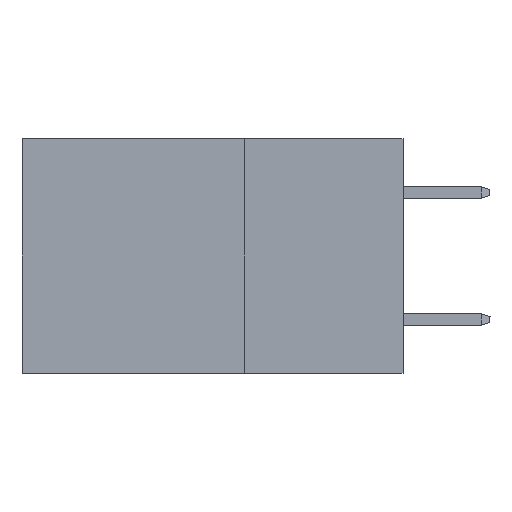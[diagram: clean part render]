
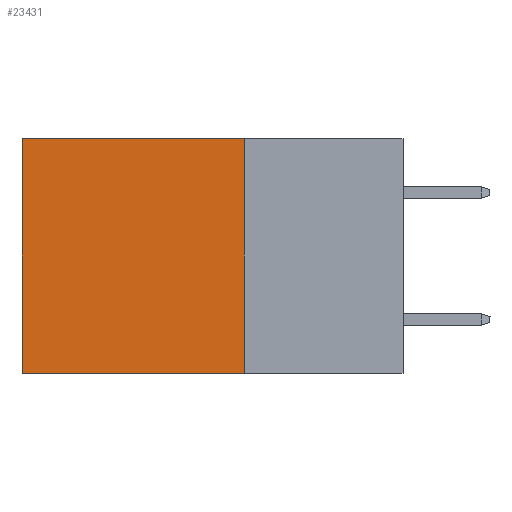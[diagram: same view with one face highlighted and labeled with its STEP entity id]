
A CAD part, left-side view. The second image highlights one B-rep face of the part: STEP entity #23431.
In plain terms, the highlighted planar face has unit normal (-1, 0, 0).
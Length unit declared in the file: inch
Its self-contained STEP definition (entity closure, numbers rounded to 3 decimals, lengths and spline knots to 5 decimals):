
#211 = ORIENTED_EDGE ( 'NONE', *, *, #19550, .T. ) ;
#2471 = DIRECTION ( 'NONE',  ( 0., 0., -1. ) ) ;
#2619 = EDGE_CURVE ( 'NONE', #22974, #35221, #35908, .T. ) ;
#2854 = ORIENTED_EDGE ( 'NONE', *, *, #12509, .F. ) ;
#3953 = VECTOR ( 'NONE', #25395, 39.37008 ) ;
#5380 = CARTESIAN_POINT ( 'NONE',  ( 0.2875, 0.25, 0. ) ) ;
#6935 = AXIS2_PLACEMENT_3D ( 'NONE', #5380, #34425, #2471 ) ;
#10075 = VECTOR ( 'NONE', #26788, 39.37008 ) ;
#11031 = VECTOR ( 'NONE', #27365, 39.37008 ) ;
#11593 = CARTESIAN_POINT ( 'NONE',  ( 0.2875, 0.6, 0. ) ) ;
#12509 = EDGE_CURVE ( 'NONE', #17245, #16819, #28801, .T. ) ;
#13419 = CARTESIAN_POINT ( 'NONE',  ( 0.2875, 0.25, -0.37 ) ) ;
#15440 = EDGE_CURVE ( 'NONE', #16819, #35221, #16892, .T. ) ;
#16173 = EDGE_LOOP ( 'NONE', ( #26280, #20005, #2854, #211 ) ) ;
#16744 = VECTOR ( 'NONE', #22013, 39.37008 ) ;
#16819 = VERTEX_POINT ( 'NONE', #34163 ) ;
#16892 = LINE ( 'NONE', #13419, #3953 ) ;
#17245 = VERTEX_POINT ( 'NONE', #30408 ) ;
#19550 = EDGE_CURVE ( 'NONE', #17245, #22974, #24629, .T. ) ;
#19689 = CARTESIAN_POINT ( 'NONE',  ( 0.2875, 0.25, 0. ) ) ;
#20005 = ORIENTED_EDGE ( 'NONE', *, *, #15440, .F. ) ;
#22013 = DIRECTION ( 'NONE',  ( 0., 0., -1. ) ) ;
#22974 = VERTEX_POINT ( 'NONE', #11593 ) ;
#23431 = ADVANCED_FACE ( 'NONE', ( #32253 ), #31871, .F. ) ;
#24629 = LINE ( 'NONE', #30830, #11031 ) ;
#25395 = DIRECTION ( 'NONE',  ( 0., 1., 0. ) ) ;
#26280 = ORIENTED_EDGE ( 'NONE', *, *, #2619, .T. ) ;
#26788 = DIRECTION ( 'NONE',  ( 0., 0., -1. ) ) ;
#27365 = DIRECTION ( 'NONE',  ( 0., 1., 0. ) ) ;
#27573 = CARTESIAN_POINT ( 'NONE',  ( 0.2875, 0.6, -0.37 ) ) ;
#28801 = LINE ( 'NONE', #19689, #16744 ) ;
#29881 = CARTESIAN_POINT ( 'NONE',  ( 0.2875, 0.6, 0. ) ) ;
#30408 = CARTESIAN_POINT ( 'NONE',  ( 0.2875, 0.25, 0. ) ) ;
#30830 = CARTESIAN_POINT ( 'NONE',  ( 0.2875, 0.25, 0. ) ) ;
#31871 = PLANE ( 'NONE',  #6935 ) ;
#32253 = FACE_OUTER_BOUND ( 'NONE', #16173, .T. ) ;
#34163 = CARTESIAN_POINT ( 'NONE',  ( 0.2875, 0.25, -0.37 ) ) ;
#34425 = DIRECTION ( 'NONE',  ( 1., 0., 0. ) ) ;
#35221 = VERTEX_POINT ( 'NONE', #27573 ) ;
#35908 = LINE ( 'NONE', #29881, #10075 ) ;
